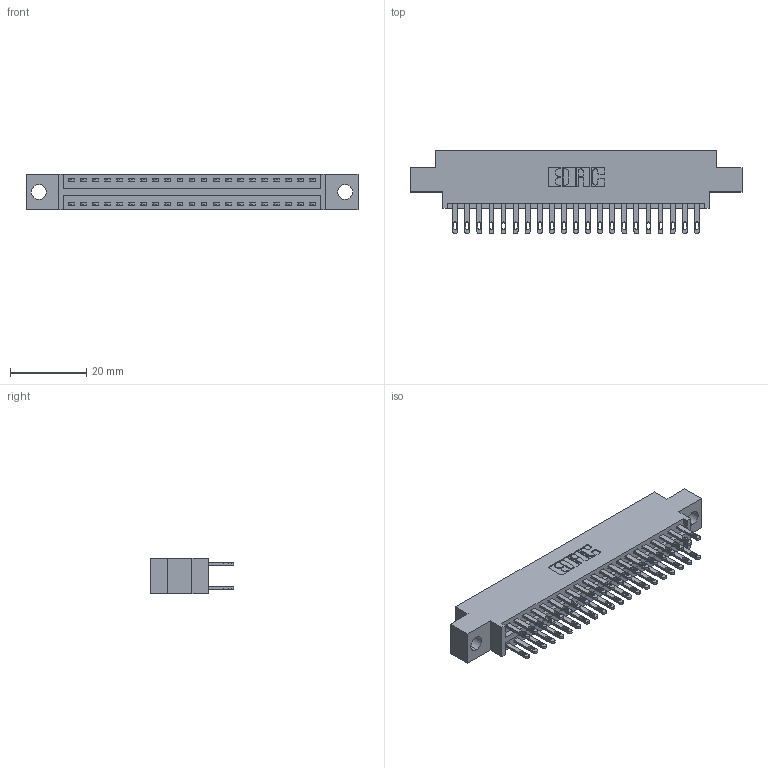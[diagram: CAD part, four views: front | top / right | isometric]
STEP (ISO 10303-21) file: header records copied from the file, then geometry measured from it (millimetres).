
FILE_DESCRIPTION (( 'STEP AP203' ), '1' );
FILE_NAME ('346-042-500-804.STEP', '2022-05-20T03:29:50', ( '' ), ( '' ), 'SwSTEP 2.0', 'SolidWorks 2020', '' );
FILE_SCHEMA (( 'CONFIG_CONTROL_DESIGN' ));
Length unit declared in the file: inch
Products named in the file (3): 346-042-500-804; 346 Part_0.170 Offset - 0.156 Dia-TH; 345-292-001_345-293-100
Assembly tree (43 placements, depth 2):
  346-042-500-804
    346 Part_0.170 Offset - 0.156 Dia-TH
    345-292-001_345-293-100  x42
Bounding box: 87.25 x 21.84 x 9.4 mm (x, y, z)
Volume: 8212.5 mm3; surface area: 11425.7 mm2
Topology: 43 solids, 43 shells, 2156 faces, 6551 edges, 4366 vertices
Faces by surface type: plane 1312, cylinder 844
Entity records: 17013 total; most frequent: CARTESIAN_POINT 2838, ORIENTED_EDGE 2770, DIRECTION 2553, EDGE_CURVE 1385, LINE 1165, VECTOR 1165, VERTEX_POINT 922, AXIS2_PLACEMENT_3D 694
